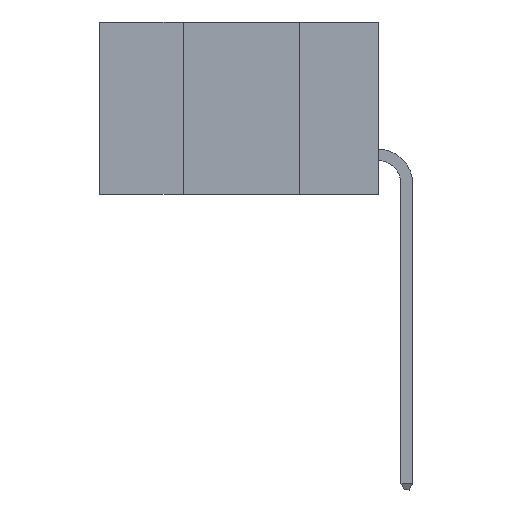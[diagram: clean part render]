
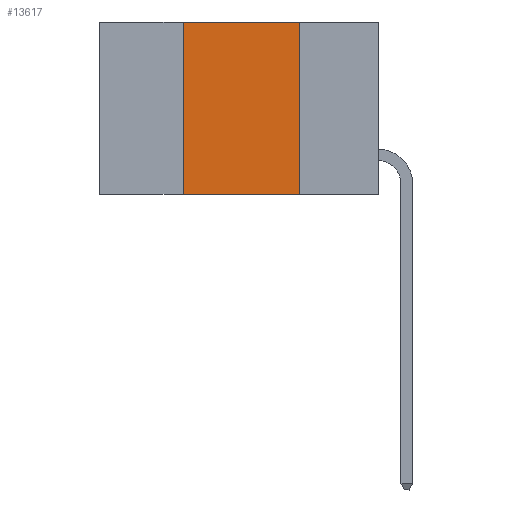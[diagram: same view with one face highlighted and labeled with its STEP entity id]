
A CAD part, left-side view. The second image highlights one B-rep face of the part: STEP entity #13617.
In plain terms, the highlighted planar face has unit normal (-1, 0, 0).
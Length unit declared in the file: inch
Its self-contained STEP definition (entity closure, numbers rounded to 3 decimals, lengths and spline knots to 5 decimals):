
#70 = ORIENTED_EDGE ( 'NONE', *, *, #4469, .T. ) ;
#1239 = VECTOR ( 'NONE', #7124, 39.37008 ) ;
#1689 = VECTOR ( 'NONE', #14118, 39.37008 ) ;
#1746 = CARTESIAN_POINT ( 'NONE',  ( 0., 0.6, -0.37 ) ) ;
#1943 = VERTEX_POINT ( 'NONE', #9769 ) ;
#2065 = EDGE_CURVE ( 'NONE', #11588, #2375, #11610, .T. ) ;
#2375 = VERTEX_POINT ( 'NONE', #4510 ) ;
#3157 = EDGE_LOOP ( 'NONE', ( #11451, #3577, #10556, #70 ) ) ;
#3394 = DIRECTION ( 'NONE',  ( 1., 0., 0. ) ) ;
#3573 = VECTOR ( 'NONE', #4848, 39.37008 ) ;
#3577 = ORIENTED_EDGE ( 'NONE', *, *, #12346, .F. ) ;
#4456 = DIRECTION ( 'NONE',  ( 0., -1., 0. ) ) ;
#4469 = EDGE_CURVE ( 'NONE', #11588, #1943, #17120, .T. ) ;
#4510 = CARTESIAN_POINT ( 'NONE',  ( 0., 0.42, 0. ) ) ;
#4848 = DIRECTION ( 'NONE',  ( 0., 0., 1. ) ) ;
#5901 = CARTESIAN_POINT ( 'NONE',  ( 0., 0.6, 0. ) ) ;
#6443 = EDGE_CURVE ( 'NONE', #7844, #1943, #12098, .T. ) ;
#7124 = DIRECTION ( 'NONE',  ( 0., 0., -1. ) ) ;
#7844 = VERTEX_POINT ( 'NONE', #8062 ) ;
#8062 = CARTESIAN_POINT ( 'NONE',  ( 0., 0.17, 0. ) ) ;
#8535 = VECTOR ( 'NONE', #4456, 39.37008 ) ;
#9045 = DIRECTION ( 'NONE',  ( 0., 0., -1. ) ) ;
#9208 = CARTESIAN_POINT ( 'NONE',  ( 0., 0.42, -0.37 ) ) ;
#9769 = CARTESIAN_POINT ( 'NONE',  ( 0., 0.17, -0.37 ) ) ;
#9778 = CARTESIAN_POINT ( 'NONE',  ( 0., 0.17, 0. ) ) ;
#10556 = ORIENTED_EDGE ( 'NONE', *, *, #2065, .F. ) ;
#11183 = FACE_OUTER_BOUND ( 'NONE', #3157, .T. ) ;
#11451 = ORIENTED_EDGE ( 'NONE', *, *, #6443, .F. ) ;
#11588 = VERTEX_POINT ( 'NONE', #9208 ) ;
#11610 = LINE ( 'NONE', #13281, #3573 ) ;
#11856 = LINE ( 'NONE', #5901, #1689 ) ;
#11866 = PLANE ( 'NONE',  #13959 ) ;
#12098 = LINE ( 'NONE', #9778, #1239 ) ;
#12346 = EDGE_CURVE ( 'NONE', #2375, #7844, #11856, .T. ) ;
#13281 = CARTESIAN_POINT ( 'NONE',  ( 0., 0.42, 0. ) ) ;
#13617 = ADVANCED_FACE ( 'NONE', ( #11183 ), #11866, .F. ) ;
#13959 = AXIS2_PLACEMENT_3D ( 'NONE', #14405, #3394, #9045 ) ;
#14118 = DIRECTION ( 'NONE',  ( 0., -1., 0. ) ) ;
#14405 = CARTESIAN_POINT ( 'NONE',  ( 0., 0.6, 0. ) ) ;
#17120 = LINE ( 'NONE', #1746, #8535 ) ;
